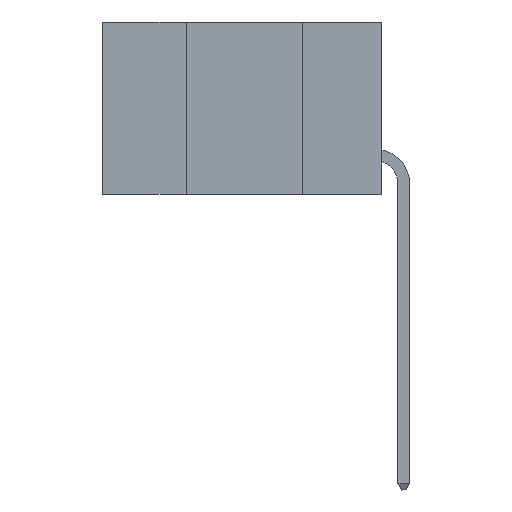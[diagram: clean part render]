
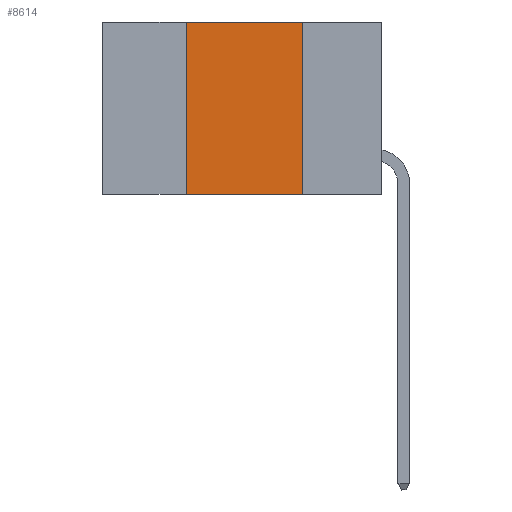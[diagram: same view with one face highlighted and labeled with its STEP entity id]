
A CAD part, left-side view. The second image highlights one B-rep face of the part: STEP entity #8614.
In plain terms, the highlighted planar face has unit normal (-1, 0, 0).
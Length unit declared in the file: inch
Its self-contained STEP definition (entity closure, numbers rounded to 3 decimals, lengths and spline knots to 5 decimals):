
#390 = FACE_OUTER_BOUND ( 'NONE', #9320, .T. ) ;
#712 = CARTESIAN_POINT ( 'NONE',  ( 0., 0.42, -0.37 ) ) ;
#865 = ORIENTED_EDGE ( 'NONE', *, *, #15591, .F. ) ;
#1385 = CARTESIAN_POINT ( 'NONE',  ( 0., 0.17, 0. ) ) ;
#1807 = DIRECTION ( 'NONE',  ( 0., -1., 0. ) ) ;
#3100 = CARTESIAN_POINT ( 'NONE',  ( 0., 0.6, 0. ) ) ;
#3254 = CARTESIAN_POINT ( 'NONE',  ( 0., 0.42, 0. ) ) ;
#4045 = CARTESIAN_POINT ( 'NONE',  ( 0., 0.17, -0.37 ) ) ;
#4683 = DIRECTION ( 'NONE',  ( 0., -1., 0. ) ) ;
#4701 = ORIENTED_EDGE ( 'NONE', *, *, #12484, .F. ) ;
#5256 = LINE ( 'NONE', #3100, #13498 ) ;
#5565 = CARTESIAN_POINT ( 'NONE',  ( 0., 0.42, 0. ) ) ;
#5841 = CARTESIAN_POINT ( 'NONE',  ( 0., 0.6, -0.37 ) ) ;
#7538 = CARTESIAN_POINT ( 'NONE',  ( 0., 0.6, 0. ) ) ;
#7660 = DIRECTION ( 'NONE',  ( 0., 0., -1. ) ) ;
#7860 = ORIENTED_EDGE ( 'NONE', *, *, #17393, .T. ) ;
#8306 = PLANE ( 'NONE',  #12784 ) ;
#8466 = LINE ( 'NONE', #5841, #16065 ) ;
#8614 = ADVANCED_FACE ( 'NONE', ( #390 ), #8306, .F. ) ;
#9320 = EDGE_LOOP ( 'NONE', ( #4701, #16885, #865, #7860 ) ) ;
#9326 = EDGE_CURVE ( 'NONE', #14931, #12236, #5256, .T. ) ;
#11940 = VERTEX_POINT ( 'NONE', #712 ) ;
#12014 = DIRECTION ( 'NONE',  ( 1., 0., 0. ) ) ;
#12236 = VERTEX_POINT ( 'NONE', #14519 ) ;
#12297 = DIRECTION ( 'NONE',  ( 0., 0., 1. ) ) ;
#12484 = EDGE_CURVE ( 'NONE', #12236, #14632, #12942, .T. ) ;
#12784 = AXIS2_PLACEMENT_3D ( 'NONE', #7538, #12014, #17470 ) ;
#12942 = LINE ( 'NONE', #1385, #13771 ) ;
#13498 = VECTOR ( 'NONE', #1807, 39.37008 ) ;
#13771 = VECTOR ( 'NONE', #7660, 39.37008 ) ;
#14483 = VECTOR ( 'NONE', #12297, 39.37008 ) ;
#14519 = CARTESIAN_POINT ( 'NONE',  ( 0., 0.17, 0. ) ) ;
#14632 = VERTEX_POINT ( 'NONE', #4045 ) ;
#14931 = VERTEX_POINT ( 'NONE', #3254 ) ;
#15591 = EDGE_CURVE ( 'NONE', #11940, #14931, #15948, .T. ) ;
#15948 = LINE ( 'NONE', #5565, #14483 ) ;
#16065 = VECTOR ( 'NONE', #4683, 39.37008 ) ;
#16885 = ORIENTED_EDGE ( 'NONE', *, *, #9326, .F. ) ;
#17393 = EDGE_CURVE ( 'NONE', #11940, #14632, #8466, .T. ) ;
#17470 = DIRECTION ( 'NONE',  ( 0., 0., -1. ) ) ;
